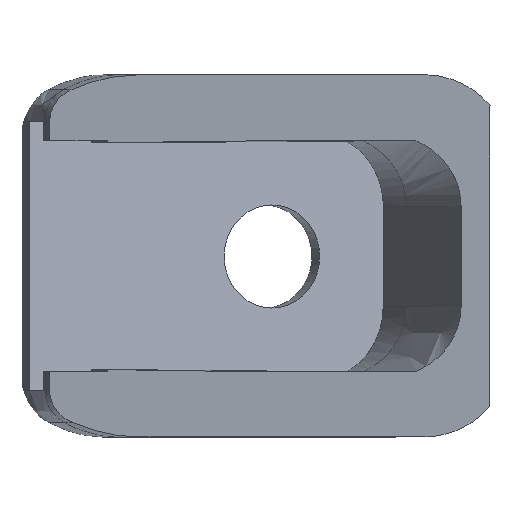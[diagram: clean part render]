
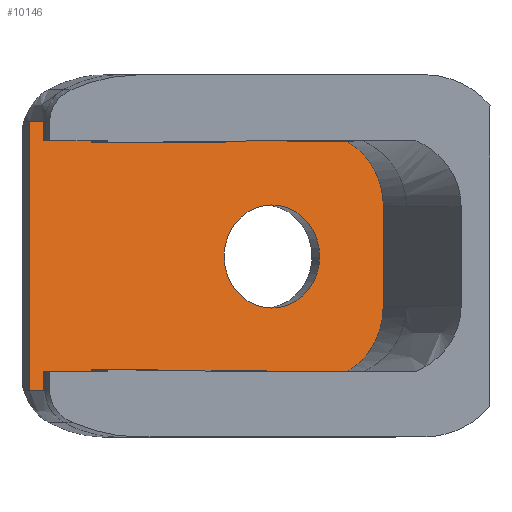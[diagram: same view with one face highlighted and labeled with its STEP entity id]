
A CAD part, top view. The second image highlights one B-rep face of the part: STEP entity #10146.
In plain terms, the highlighted planar face has unit normal (0.376, 0, 0.927).
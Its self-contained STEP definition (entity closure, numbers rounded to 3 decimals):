
#89=FACE_BOUND('',#1574,.T.);
#524=PLANE('',#10723);
#1014=FACE_OUTER_BOUND('',#1573,.T.);
#1573=EDGE_LOOP('',(#9331,#9332,#9333,#9334,#9335,#9336,#9337,#9338,#9339,
#9340,#9341,#9342));
#1574=EDGE_LOOP('',(#9343));
#1747=B_SPLINE_CURVE_WITH_KNOTS('',3,(#22042,#22043,#22044,#22045),
 .UNSPECIFIED.,.F.,.F.,(4,4),(-0.389,-0.389),
 .UNSPECIFIED.);
#1753=B_SPLINE_CURVE_WITH_KNOTS('',3,(#22150,#22151,#22152,#22153),
 .UNSPECIFIED.,.F.,.F.,(4,4),(-0.008,0.),.UNSPECIFIED.);
#1754=B_SPLINE_CURVE_WITH_KNOTS('',3,(#22161,#22162,#22163,#22164,#22165,
#22166,#22167,#22168,#22169,#22170,#22171,#22172,#22173,#22174,#22175,#22176),
 .UNSPECIFIED.,.F.,.F.,(4,3,3,3,3,4),(-0.527,-0.434,
-0.338,-0.178,-0.021,0.),
 .UNSPECIFIED.);
#1755=B_SPLINE_CURVE_WITH_KNOTS('',3,(#22180,#22181,#22182,#22183,#22184,
#22185,#22186,#22187,#22188,#22189,#22190,#22191,#22192,#22193,#22194,#22195),
 .UNSPECIFIED.,.F.,.F.,(4,3,3,3,3,4),(-1.134,-1.088,
-0.909,-0.72,-0.365,0.),
 .UNSPECIFIED.);
#2978=LINE('',#22148,#4211);
#2979=LINE('',#22155,#4212);
#2980=LINE('',#22157,#4213);
#2981=LINE('',#22178,#4214);
#2982=LINE('',#22199,#4215);
#2983=LINE('',#22200,#4216);
#4211=VECTOR('',#12957,10.);
#4212=VECTOR('',#12958,10.);
#4213=VECTOR('',#12959,10.);
#4214=VECTOR('',#12962,10.);
#4215=VECTOR('',#12965,10.);
#4216=VECTOR('',#12966,10.);
#4307=CIRCLE('',#10724,943.89);
#4308=CIRCLE('',#10725,943.89);
#4309=CIRCLE('',#10726,5.);
#5201=VERTEX_POINT('',#22036);
#5202=VERTEX_POINT('',#22041);
#5223=VERTEX_POINT('',#22147);
#5224=VERTEX_POINT('',#22149);
#5225=VERTEX_POINT('',#22154);
#5226=VERTEX_POINT('',#22156);
#5227=VERTEX_POINT('',#22158);
#5228=VERTEX_POINT('',#22160);
#5229=VERTEX_POINT('',#22177);
#5230=VERTEX_POINT('',#22179);
#5231=VERTEX_POINT('',#22196);
#5232=VERTEX_POINT('',#22198);
#5233=VERTEX_POINT('',#22201);
#6606=EDGE_CURVE('',#5201,#5202,#1747,.T.);
#6629=EDGE_CURVE('',#5223,#5201,#2978,.T.);
#6630=EDGE_CURVE('',#5224,#5223,#1753,.T.);
#6631=EDGE_CURVE('',#5224,#5225,#2979,.F.);
#6632=EDGE_CURVE('',#5225,#5226,#2980,.T.);
#6633=EDGE_CURVE('',#5227,#5226,#4307,.T.);
#6634=EDGE_CURVE('',#5228,#5227,#1754,.T.);
#6635=EDGE_CURVE('',#5229,#5228,#2981,.T.);
#6636=EDGE_CURVE('',#5230,#5229,#1755,.T.);
#6637=EDGE_CURVE('',#5231,#5230,#4308,.T.);
#6638=EDGE_CURVE('',#5231,#5232,#2982,.T.);
#6639=EDGE_CURVE('',#5202,#5232,#2983,.T.);
#6640=EDGE_CURVE('',#5233,#5233,#4309,.T.);
#9331=ORIENTED_EDGE('',*,*,#6606,.F.);
#9332=ORIENTED_EDGE('',*,*,#6629,.F.);
#9333=ORIENTED_EDGE('',*,*,#6630,.F.);
#9334=ORIENTED_EDGE('',*,*,#6631,.T.);
#9335=ORIENTED_EDGE('',*,*,#6632,.T.);
#9336=ORIENTED_EDGE('',*,*,#6633,.F.);
#9337=ORIENTED_EDGE('',*,*,#6634,.F.);
#9338=ORIENTED_EDGE('',*,*,#6635,.F.);
#9339=ORIENTED_EDGE('',*,*,#6636,.F.);
#9340=ORIENTED_EDGE('',*,*,#6637,.F.);
#9341=ORIENTED_EDGE('',*,*,#6638,.T.);
#9342=ORIENTED_EDGE('',*,*,#6639,.F.);
#9343=ORIENTED_EDGE('',*,*,#6640,.T.);
#10146=ADVANCED_FACE('',(#1014,#89),#524,.F.);
#10723=AXIS2_PLACEMENT_3D('',#22146,#12955,#12956);
#10724=AXIS2_PLACEMENT_3D('',#22159,#12960,#12961);
#10725=AXIS2_PLACEMENT_3D('',#22197,#12963,#12964);
#10726=AXIS2_PLACEMENT_3D('',#22202,#12967,#12968);
#12955=DIRECTION('center_axis',(-0.376,0.,
-0.927));
#12956=DIRECTION('ref_axis',(-0.927,0.,0.376));
#12957=DIRECTION('',(0.,1.,0.));
#12958=DIRECTION('',(-0.927,0.,0.376));
#12959=DIRECTION('',(0.,1.,0.));
#12960=DIRECTION('center_axis',(-0.376,0.,
-0.927));
#12961=DIRECTION('ref_axis',(0.005,-1.,-0.002));
#12962=DIRECTION('',(0.,-1.,0.));
#12963=DIRECTION('center_axis',(-0.376,0.,
-0.927));
#12964=DIRECTION('ref_axis',(-0.023,1.,0.009));
#12965=DIRECTION('',(0.,1.,0.));
#12966=DIRECTION('',(0.927,0.,-0.376));
#12967=DIRECTION('center_axis',(-0.376,0.,
-0.927));
#12968=DIRECTION('ref_axis',(0.,-1.,0.));
#22036=CARTESIAN_POINT('',(45.289,35.663,18.677));
#22041=CARTESIAN_POINT('',(45.289,35.666,18.677));
#22042=CARTESIAN_POINT('Ctrl Pts',(45.289,35.663,18.677));
#22043=CARTESIAN_POINT('Ctrl Pts',(45.289,35.664,18.677));
#22044=CARTESIAN_POINT('Ctrl Pts',(45.289,35.665,18.677));
#22045=CARTESIAN_POINT('Ctrl Pts',(45.289,35.666,18.677));
#22146=CARTESIAN_POINT('Origin',(61.252,22.61,12.204));
#22147=CARTESIAN_POINT('',(45.289,9.63,18.677));
#22148=CARTESIAN_POINT('',(45.289,15.144,18.677));
#22149=CARTESIAN_POINT('',(45.29,9.555,18.677));
#22150=CARTESIAN_POINT('Ctrl Pts',(45.29,9.555,18.677));
#22151=CARTESIAN_POINT('Ctrl Pts',(45.289,9.58,18.677));
#22152=CARTESIAN_POINT('Ctrl Pts',(45.289,9.605,18.677));
#22153=CARTESIAN_POINT('Ctrl Pts',(45.289,9.63,18.677));
#22154=CARTESIAN_POINT('',(49.922,9.555,16.798));
#22155=CARTESIAN_POINT('',(53.271,9.555,15.44));
#22156=CARTESIAN_POINT('',(49.922,9.768,16.798));
#22157=CARTESIAN_POINT('',(49.922,22.61,16.798));
#22158=CARTESIAN_POINT('',(74.21,9.555,6.949));
#22159=CARTESIAN_POINT('Origin',(69.176,953.429,8.991));
#22160=CARTESIAN_POINT('',(79.691,17.789,4.727));
#22161=CARTESIAN_POINT('Ctrl Pts',(79.691,17.789,4.727));
#22162=CARTESIAN_POINT('Ctrl Pts',(79.691,17.153,4.727));
#22163=CARTESIAN_POINT('Ctrl Pts',(79.627,16.519,4.752));
#22164=CARTESIAN_POINT('Ctrl Pts',(79.501,15.897,4.803));
#22165=CARTESIAN_POINT('Ctrl Pts',(79.37,15.248,4.857));
#22166=CARTESIAN_POINT('Ctrl Pts',(79.171,14.616,4.938));
#22167=CARTESIAN_POINT('Ctrl Pts',(78.906,14.014,5.045));
#22168=CARTESIAN_POINT('Ctrl Pts',(78.468,13.016,5.223));
#22169=CARTESIAN_POINT('Ctrl Pts',(77.855,12.111,5.471));
#22170=CARTESIAN_POINT('Ctrl Pts',(77.092,11.358,5.78));
#22171=CARTESIAN_POINT('Ctrl Pts',(76.346,10.621,6.083));
#22172=CARTESIAN_POINT('Ctrl Pts',(75.469,10.044,6.438));
#22173=CARTESIAN_POINT('Ctrl Pts',(74.508,9.671,6.828));
#22174=CARTESIAN_POINT('Ctrl Pts',(74.409,9.632,6.869));
#22175=CARTESIAN_POINT('Ctrl Pts',(74.309,9.594,6.909));
#22176=CARTESIAN_POINT('Ctrl Pts',(74.21,9.555,6.949));
#22177=CARTESIAN_POINT('',(79.691,27.432,4.727));
#22178=CARTESIAN_POINT('',(79.691,20.2,4.727));
#22179=CARTESIAN_POINT('',(74.21,35.666,6.949));
#22180=CARTESIAN_POINT('Ctrl Pts',(74.21,35.666,6.949));
#22181=CARTESIAN_POINT('Ctrl Pts',(74.309,35.627,6.909));
#22182=CARTESIAN_POINT('Ctrl Pts',(74.409,35.588,6.869));
#22183=CARTESIAN_POINT('Ctrl Pts',(74.508,35.55,6.828));
#22184=CARTESIAN_POINT('Ctrl Pts',(75.02,35.351,6.621));
#22185=CARTESIAN_POINT('Ctrl Pts',(75.509,35.095,6.423));
#22186=CARTESIAN_POINT('Ctrl Pts',(75.967,34.785,6.237));
#22187=CARTESIAN_POINT('Ctrl Pts',(76.45,34.46,6.041));
#22188=CARTESIAN_POINT('Ctrl Pts',(76.897,34.079,5.86));
#22189=CARTESIAN_POINT('Ctrl Pts',(77.3,33.65,5.696));
#22190=CARTESIAN_POINT('Ctrl Pts',(78.06,32.843,5.388));
#22191=CARTESIAN_POINT('Ctrl Pts',(78.655,31.882,5.147));
#22192=CARTESIAN_POINT('Ctrl Pts',(79.062,30.83,4.982));
#22193=CARTESIAN_POINT('Ctrl Pts',(79.479,29.752,4.813));
#22194=CARTESIAN_POINT('Ctrl Pts',(79.691,28.596,4.727));
#22195=CARTESIAN_POINT('Ctrl Pts',(79.691,27.432,4.727));
#22196=CARTESIAN_POINT('',(49.922,35.453,16.798));
#22197=CARTESIAN_POINT('Origin',(69.176,-908.208,8.991));
#22198=CARTESIAN_POINT('',(49.922,35.666,16.798));
#22199=CARTESIAN_POINT('',(49.922,22.61,16.798));
#22200=CARTESIAN_POINT('',(53.271,35.666,15.44));
#22201=CARTESIAN_POINT('',(68.773,27.61,9.154));
#22202=CARTESIAN_POINT('Origin',(68.773,22.61,9.154));
